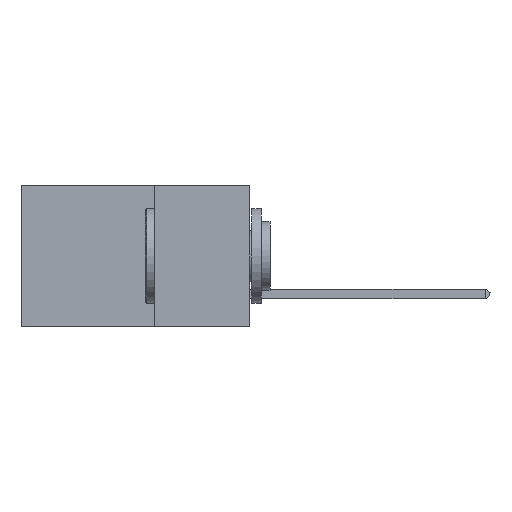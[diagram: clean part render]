
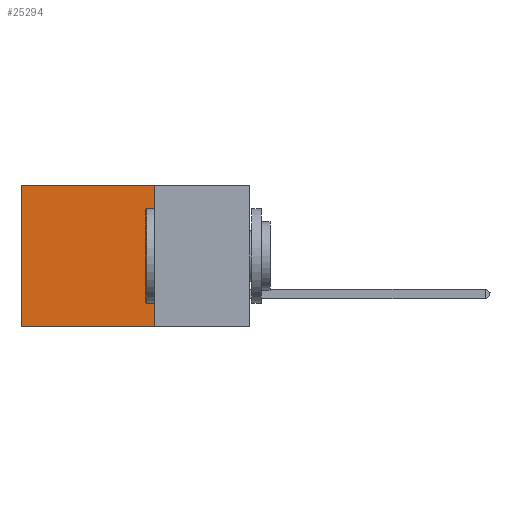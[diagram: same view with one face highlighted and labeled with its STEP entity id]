
A CAD part, left-side view. The second image highlights one B-rep face of the part: STEP entity #25294.
In plain terms, the highlighted planar face has unit normal (-1, 0, 0).
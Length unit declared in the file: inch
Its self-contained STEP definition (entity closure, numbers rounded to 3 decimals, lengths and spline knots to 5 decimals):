
#334 = CARTESIAN_POINT ( 'NONE',  ( 0.2875, 0.25, -0.37 ) ) ;
#1573 = DIRECTION ( 'NONE',  ( 0., 0., -1. ) ) ;
#3000 = FACE_OUTER_BOUND ( 'NONE', #3135, .T. ) ;
#3135 = EDGE_LOOP ( 'NONE', ( #7159, #15952, #34260, #23566 ) ) ;
#3623 = DIRECTION ( 'NONE',  ( 0., 0., -1. ) ) ;
#5262 = VECTOR ( 'NONE', #3623, 39.37008 ) ;
#7159 = ORIENTED_EDGE ( 'NONE', *, *, #38670, .T. ) ;
#8584 = VERTEX_POINT ( 'NONE', #22846 ) ;
#9438 = DIRECTION ( 'NONE',  ( 0., 1., 0. ) ) ;
#11205 = VECTOR ( 'NONE', #39071, 39.37008 ) ;
#12431 = EDGE_CURVE ( 'NONE', #28414, #37998, #23327, .T. ) ;
#12444 = AXIS2_PLACEMENT_3D ( 'NONE', #20201, #26521, #23235 ) ;
#14507 = PLANE ( 'NONE',  #12444 ) ;
#15952 = ORIENTED_EDGE ( 'NONE', *, *, #12431, .F. ) ;
#16152 = LINE ( 'NONE', #37534, #34101 ) ;
#19298 = VERTEX_POINT ( 'NONE', #38260 ) ;
#20201 = CARTESIAN_POINT ( 'NONE',  ( 0.2875, 0.25, 0. ) ) ;
#20670 = EDGE_CURVE ( 'NONE', #19298, #28414, #16152, .T. ) ;
#21326 = LINE ( 'NONE', #27490, #5262 ) ;
#22846 = CARTESIAN_POINT ( 'NONE',  ( 0.2875, 0.6, 0. ) ) ;
#23235 = DIRECTION ( 'NONE',  ( 0., 0., -1. ) ) ;
#23327 = LINE ( 'NONE', #334, #24264 ) ;
#23566 = ORIENTED_EDGE ( 'NONE', *, *, #34945, .T. ) ;
#24264 = VECTOR ( 'NONE', #9438, 39.37008 ) ;
#25294 = ADVANCED_FACE ( 'NONE', ( #3000 ), #14507, .F. ) ;
#26521 = DIRECTION ( 'NONE',  ( 1., 0., 0. ) ) ;
#26792 = CARTESIAN_POINT ( 'NONE',  ( 0.2875, 0.25, 0. ) ) ;
#27490 = CARTESIAN_POINT ( 'NONE',  ( 0.2875, 0.6, 0. ) ) ;
#27740 = LINE ( 'NONE', #26792, #11205 ) ;
#28414 = VERTEX_POINT ( 'NONE', #38069 ) ;
#34101 = VECTOR ( 'NONE', #1573, 39.37008 ) ;
#34260 = ORIENTED_EDGE ( 'NONE', *, *, #20670, .F. ) ;
#34945 = EDGE_CURVE ( 'NONE', #19298, #8584, #27740, .T. ) ;
#37148 = CARTESIAN_POINT ( 'NONE',  ( 0.2875, 0.6, -0.37 ) ) ;
#37534 = CARTESIAN_POINT ( 'NONE',  ( 0.2875, 0.25, 0. ) ) ;
#37998 = VERTEX_POINT ( 'NONE', #37148 ) ;
#38069 = CARTESIAN_POINT ( 'NONE',  ( 0.2875, 0.25, -0.37 ) ) ;
#38260 = CARTESIAN_POINT ( 'NONE',  ( 0.2875, 0.25, 0. ) ) ;
#38670 = EDGE_CURVE ( 'NONE', #8584, #37998, #21326, .T. ) ;
#39071 = DIRECTION ( 'NONE',  ( 0., 1., 0. ) ) ;
